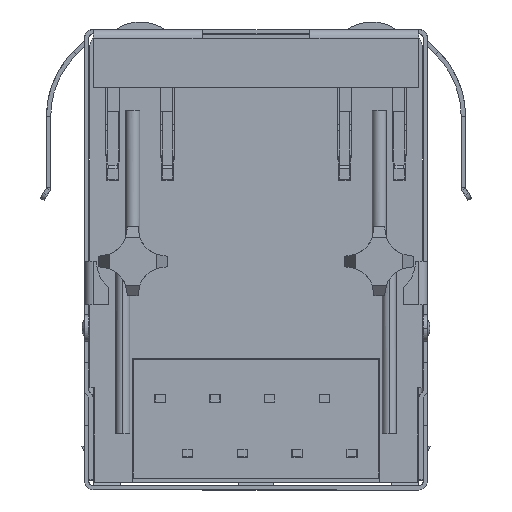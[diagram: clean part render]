
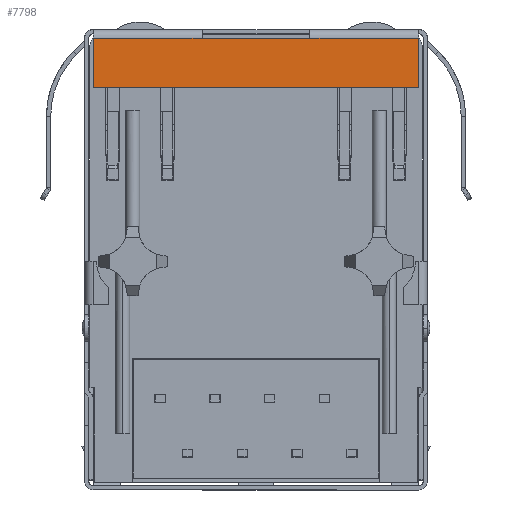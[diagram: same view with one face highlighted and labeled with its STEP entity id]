
A CAD part, front view. The second image highlights one B-rep face of the part: STEP entity #7798.
In plain terms, the highlighted planar face has unit normal (0, -1, 0).
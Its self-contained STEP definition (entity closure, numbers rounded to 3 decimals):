
#1077 = VERTEX_POINT ( 'NONE', #18789 ) ;
#2941 = LINE ( 'NONE', #6508, #42624 ) ;
#3743 = ORIENTED_EDGE ( 'NONE', *, *, #43878, .F. ) ;
#5803 = EDGE_CURVE ( 'NONE', #14833, #1077, #34399, .T. ) ;
#6322 = ORIENTED_EDGE ( 'NONE', *, *, #40870, .T. ) ;
#6508 = CARTESIAN_POINT ( 'NONE',  ( -40.474, -1.825, 9.925 ) ) ;
#6517 = LINE ( 'NONE', #47399, #17015 ) ;
#7018 = DIRECTION ( 'NONE',  ( 1., 0., 0. ) ) ;
#7231 = FACE_OUTER_BOUND ( 'NONE', #10273, .T. ) ;
#7798 = ADVANCED_FACE ( 'NONE', ( #7231 ), #33247, .T. ) ;
#8326 = CARTESIAN_POINT ( 'NONE',  ( -25.374, -1.825, 7.625 ) ) ;
#8796 = LINE ( 'NONE', #11221, #15880 ) ;
#10241 = DIRECTION ( 'NONE',  ( 1., 0., 0. ) ) ;
#10273 = EDGE_LOOP ( 'NONE', ( #3743, #6322, #44967, #23991, #15679, #24092 ) ) ;
#10400 = CARTESIAN_POINT ( 'NONE',  ( -40.474, -1.825, 10.325 ) ) ;
#11221 = CARTESIAN_POINT ( 'NONE',  ( -40.474, -1.825, 10.325 ) ) ;
#13864 = CARTESIAN_POINT ( 'NONE',  ( -30.424, -1.825, 9.925 ) ) ;
#14833 = VERTEX_POINT ( 'NONE', #8326 ) ;
#15494 = VERTEX_POINT ( 'NONE', #19042 ) ;
#15679 = ORIENTED_EDGE ( 'NONE', *, *, #41714, .F. ) ;
#15880 = VECTOR ( 'NONE', #22499, 1000. ) ;
#16579 = VERTEX_POINT ( 'NONE', #40914 ) ;
#17015 = VECTOR ( 'NONE', #36516, 1000. ) ;
#18269 = DIRECTION ( 'NONE',  ( 0., -1., 0. ) ) ;
#18789 = CARTESIAN_POINT ( 'NONE',  ( -25.374, -1.825, 9.925 ) ) ;
#19042 = CARTESIAN_POINT ( 'NONE',  ( -40.474, -1.825, 7.625 ) ) ;
#20236 = VERTEX_POINT ( 'NONE', #30830 ) ;
#21757 = DIRECTION ( 'NONE',  ( -1., 0., 0. ) ) ;
#22404 = CARTESIAN_POINT ( 'NONE',  ( -40.474, -1.825, 7.625 ) ) ;
#22499 = DIRECTION ( 'NONE',  ( 0., 0., -1. ) ) ;
#23540 = VECTOR ( 'NONE', #7018, 1000. ) ;
#23991 = ORIENTED_EDGE ( 'NONE', *, *, #5803, .T. ) ;
#24092 = ORIENTED_EDGE ( 'NONE', *, *, #44850, .T. ) ;
#28816 = CARTESIAN_POINT ( 'NONE',  ( -25.374, -1.825, 10.325 ) ) ;
#29832 = VECTOR ( 'NONE', #32206, 1000. ) ;
#30830 = CARTESIAN_POINT ( 'NONE',  ( -40.474, -1.825, 9.925 ) ) ;
#31143 = LINE ( 'NONE', #22404, #23540 ) ;
#32206 = DIRECTION ( 'NONE',  ( 1., 0., 0. ) ) ;
#33247 = PLANE ( 'NONE',  #36817 ) ;
#34399 = LINE ( 'NONE', #28816, #41927 ) ;
#34514 = LINE ( 'NONE', #40157, #29832 ) ;
#35938 = VERTEX_POINT ( 'NONE', #13864 ) ;
#36126 = DIRECTION ( 'NONE',  ( 0., 0., 1. ) ) ;
#36516 = DIRECTION ( 'NONE',  ( 1., 0., 0. ) ) ;
#36817 = AXIS2_PLACEMENT_3D ( 'NONE', #10400, #18269, #10241 ) ;
#39448 = EDGE_CURVE ( 'NONE', #15494, #14833, #31143, .T. ) ;
#40157 = CARTESIAN_POINT ( 'NONE',  ( -25.374, -1.825, 9.925 ) ) ;
#40870 = EDGE_CURVE ( 'NONE', #20236, #15494, #8796, .T. ) ;
#40914 = CARTESIAN_POINT ( 'NONE',  ( -35.424, -1.825, 9.925 ) ) ;
#41714 = EDGE_CURVE ( 'NONE', #35938, #1077, #34514, .T. ) ;
#41927 = VECTOR ( 'NONE', #36126, 1000. ) ;
#42624 = VECTOR ( 'NONE', #21757, 1000. ) ;
#43878 = EDGE_CURVE ( 'NONE', #20236, #16579, #6517, .T. ) ;
#44850 = EDGE_CURVE ( 'NONE', #35938, #16579, #2941, .T. ) ;
#44967 = ORIENTED_EDGE ( 'NONE', *, *, #39448, .T. ) ;
#47399 = CARTESIAN_POINT ( 'NONE',  ( -25.374, -1.825, 9.925 ) ) ;
